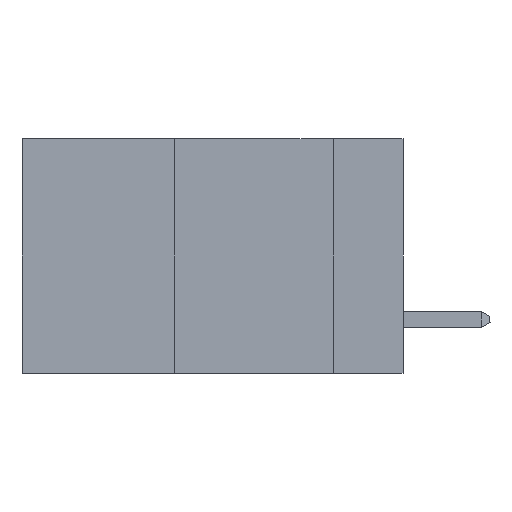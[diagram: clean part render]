
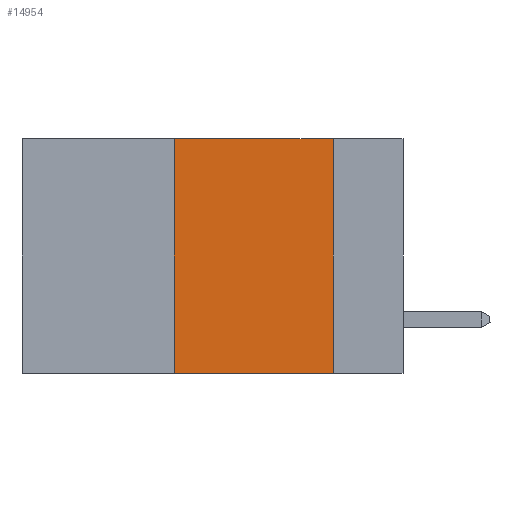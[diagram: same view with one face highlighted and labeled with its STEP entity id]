
A CAD part, left-side view. The second image highlights one B-rep face of the part: STEP entity #14954.
In plain terms, the highlighted planar face has unit normal (-1, 0, 0).
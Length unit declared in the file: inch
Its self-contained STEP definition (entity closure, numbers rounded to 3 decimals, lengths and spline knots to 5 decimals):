
#923 = CARTESIAN_POINT ( 'NONE',  ( 0., 0.6, 0. ) ) ;
#1627 = LINE ( 'NONE', #923, #5381 ) ;
#1838 = AXIS2_PLACEMENT_3D ( 'NONE', #14202, #10099, #9978 ) ;
#2907 = CARTESIAN_POINT ( 'NONE',  ( 0., 0.6, -0.37 ) ) ;
#3860 = VERTEX_POINT ( 'NONE', #8591 ) ;
#4288 = PLANE ( 'NONE',  #1838 ) ;
#5103 = CARTESIAN_POINT ( 'NONE',  ( 0., 0.36, 0. ) ) ;
#5381 = VECTOR ( 'NONE', #13592, 39.37008 ) ;
#6171 = CARTESIAN_POINT ( 'NONE',  ( 0., 0.36, -0.37 ) ) ;
#6204 = VERTEX_POINT ( 'NONE', #8272 ) ;
#6911 = EDGE_CURVE ( 'NONE', #12390, #6204, #10681, .T. ) ;
#8272 = CARTESIAN_POINT ( 'NONE',  ( 0., 0.36, 0. ) ) ;
#8426 = FACE_OUTER_BOUND ( 'NONE', #8543, .T. ) ;
#8543 = EDGE_LOOP ( 'NONE', ( #11161, #16599, #8874, #11380 ) ) ;
#8591 = CARTESIAN_POINT ( 'NONE',  ( 0., 0.11, 0. ) ) ;
#8874 = ORIENTED_EDGE ( 'NONE', *, *, #6911, .F. ) ;
#8878 = EDGE_CURVE ( 'NONE', #6204, #3860, #1627, .T. ) ;
#9978 = DIRECTION ( 'NONE',  ( 0., 0., -1. ) ) ;
#10099 = DIRECTION ( 'NONE',  ( 1., 0., 0. ) ) ;
#10681 = LINE ( 'NONE', #5103, #17945 ) ;
#11161 = ORIENTED_EDGE ( 'NONE', *, *, #17136, .F. ) ;
#11375 = CARTESIAN_POINT ( 'NONE',  ( 0., 0.11, 0. ) ) ;
#11380 = ORIENTED_EDGE ( 'NONE', *, *, #14633, .T. ) ;
#12109 = VECTOR ( 'NONE', #14804, 39.37008 ) ;
#12390 = VERTEX_POINT ( 'NONE', #6171 ) ;
#13592 = DIRECTION ( 'NONE',  ( 0., -1., 0. ) ) ;
#14202 = CARTESIAN_POINT ( 'NONE',  ( 0., 0.6, 0. ) ) ;
#14492 = CARTESIAN_POINT ( 'NONE',  ( 0., 0.11, -0.37 ) ) ;
#14633 = EDGE_CURVE ( 'NONE', #12390, #18113, #14766, .T. ) ;
#14766 = LINE ( 'NONE', #2907, #18095 ) ;
#14804 = DIRECTION ( 'NONE',  ( 0., 0., -1. ) ) ;
#14818 = DIRECTION ( 'NONE',  ( 0., 0., 1. ) ) ;
#14925 = LINE ( 'NONE', #11375, #12109 ) ;
#14954 = ADVANCED_FACE ( 'NONE', ( #8426 ), #4288, .F. ) ;
#16070 = DIRECTION ( 'NONE',  ( 0., -1., 0. ) ) ;
#16599 = ORIENTED_EDGE ( 'NONE', *, *, #8878, .F. ) ;
#17136 = EDGE_CURVE ( 'NONE', #3860, #18113, #14925, .T. ) ;
#17945 = VECTOR ( 'NONE', #14818, 39.37008 ) ;
#18095 = VECTOR ( 'NONE', #16070, 39.37008 ) ;
#18113 = VERTEX_POINT ( 'NONE', #14492 ) ;
